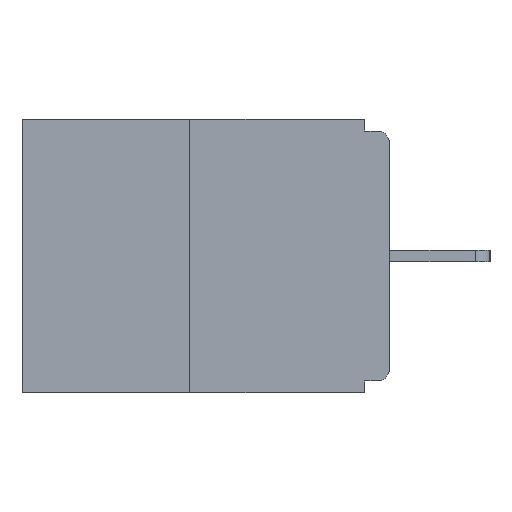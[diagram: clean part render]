
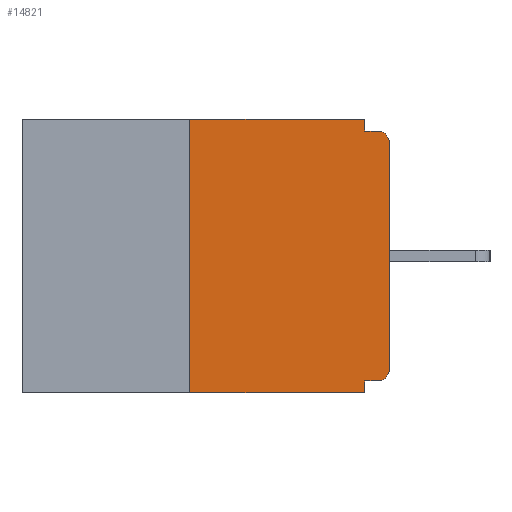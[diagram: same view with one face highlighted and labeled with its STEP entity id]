
A CAD part, left-side view. The second image highlights one B-rep face of the part: STEP entity #14821.
In plain terms, the highlighted planar face has unit normal (-1, 0, 0).
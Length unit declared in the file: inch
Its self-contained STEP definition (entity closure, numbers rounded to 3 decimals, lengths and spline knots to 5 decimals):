
#307 = VECTOR ( 'NONE', #3130, 39.37008 ) ;
#328 = LINE ( 'NONE', #7674, #12942 ) ;
#550 = DIRECTION ( 'NONE',  ( 1., 0., 0. ) ) ;
#706 = CARTESIAN_POINT ( 'NONE',  ( 0., 0.015, -0.015 ) ) ;
#743 = CIRCLE ( 'NONE', #5859, 0.015 ) ;
#1013 = VECTOR ( 'NONE', #22532, 39.37008 ) ;
#1101 = CARTESIAN_POINT ( 'NONE',  ( 0., 0., -0.03 ) ) ;
#1114 = DIRECTION ( 'NONE',  ( 0., 0., -1. ) ) ;
#1404 = CARTESIAN_POINT ( 'NONE',  ( 0., 0., -0.015 ) ) ;
#1560 = ORIENTED_EDGE ( 'NONE', *, *, #10027, .F. ) ;
#1850 = ORIENTED_EDGE ( 'NONE', *, *, #3985, .T. ) ;
#1979 = CARTESIAN_POINT ( 'NONE',  ( 0., 0.031, 0. ) ) ;
#2282 = CARTESIAN_POINT ( 'NONE',  ( 0., 0.46, 0. ) ) ;
#3026 = DIRECTION ( 'NONE',  ( 0., 0., -1. ) ) ;
#3130 = DIRECTION ( 'NONE',  ( 0., -1., 0. ) ) ;
#3823 = CIRCLE ( 'NONE', #12956, 0.015 ) ;
#3985 = EDGE_CURVE ( 'NONE', #8892, #7891, #743, .T. ) ;
#4742 = LINE ( 'NONE', #1404, #307 ) ;
#5058 = DIRECTION ( 'NONE',  ( 0., 0., 1. ) ) ;
#5859 = AXIS2_PLACEMENT_3D ( 'NONE', #19344, #10305, #22446 ) ;
#6465 = DIRECTION ( 'NONE',  ( 0., 0., -1. ) ) ;
#6553 = ORIENTED_EDGE ( 'NONE', *, *, #10595, .F. ) ;
#6658 = VERTEX_POINT ( 'NONE', #10700 ) ;
#7321 = EDGE_CURVE ( 'NONE', #12602, #14722, #8592, .T. ) ;
#7337 = CARTESIAN_POINT ( 'NONE',  ( 0., 0.031, 0. ) ) ;
#7428 = VECTOR ( 'NONE', #3026, 39.37008 ) ;
#7550 = ORIENTED_EDGE ( 'NONE', *, *, #7321, .T. ) ;
#7651 = EDGE_CURVE ( 'NONE', #12077, #7891, #4742, .T. ) ;
#7674 = CARTESIAN_POINT ( 'NONE',  ( 0., 0.46, 0. ) ) ;
#7891 = VERTEX_POINT ( 'NONE', #706 ) ;
#8220 = VERTEX_POINT ( 'NONE', #14110 ) ;
#8357 = CARTESIAN_POINT ( 'NONE',  ( 0., 0.46, -0.343 ) ) ;
#8382 = ORIENTED_EDGE ( 'NONE', *, *, #22657, .T. ) ;
#8491 = ORIENTED_EDGE ( 'NONE', *, *, #7651, .F. ) ;
#8592 = LINE ( 'NONE', #8357, #1013 ) ;
#8892 = VERTEX_POINT ( 'NONE', #1101 ) ;
#9675 = LINE ( 'NONE', #14958, #7428 ) ;
#9710 = DIRECTION ( 'NONE',  ( 0., 0., -1. ) ) ;
#9951 = LINE ( 'NONE', #17312, #18671 ) ;
#10015 = ORIENTED_EDGE ( 'NONE', *, *, #22618, .F. ) ;
#10027 = EDGE_CURVE ( 'NONE', #10649, #14722, #9675, .T. ) ;
#10154 = CARTESIAN_POINT ( 'NONE',  ( 0., 0.25, -0.343 ) ) ;
#10305 = DIRECTION ( 'NONE',  ( -1., 0., 0. ) ) ;
#10595 = EDGE_CURVE ( 'NONE', #6658, #10649, #20749, .T. ) ;
#10649 = VERTEX_POINT ( 'NONE', #17084 ) ;
#10700 = CARTESIAN_POINT ( 'NONE',  ( 0., 0.015, -0.328 ) ) ;
#10986 = FACE_OUTER_BOUND ( 'NONE', #12770, .T. ) ;
#11115 = DIRECTION ( 'NONE',  ( 0., -1., 0. ) ) ;
#11695 = DIRECTION ( 'NONE',  ( 0., 1., 0. ) ) ;
#12077 = VERTEX_POINT ( 'NONE', #16831 ) ;
#12139 = DIRECTION ( 'NONE',  ( 0., 0., 1. ) ) ;
#12190 = EDGE_CURVE ( 'NONE', #12602, #8220, #9951, .T. ) ;
#12298 = ORIENTED_EDGE ( 'NONE', *, *, #17455, .T. ) ;
#12602 = VERTEX_POINT ( 'NONE', #10154 ) ;
#12770 = EDGE_LOOP ( 'NONE', ( #10015, #16551, #7550, #1560, #6553, #8382, #12298, #1850, #8491, #15523 ) ) ;
#12928 = VECTOR ( 'NONE', #6465, 39.37008 ) ;
#12942 = VECTOR ( 'NONE', #11115, 39.37008 ) ;
#12956 = AXIS2_PLACEMENT_3D ( 'NONE', #14787, #18437, #9710 ) ;
#13066 = AXIS2_PLACEMENT_3D ( 'NONE', #2282, #550, #1114 ) ;
#13228 = VERTEX_POINT ( 'NONE', #19649 ) ;
#13278 = VECTOR ( 'NONE', #11695, 39.37008 ) ;
#14110 = CARTESIAN_POINT ( 'NONE',  ( 0., 0.25, 0. ) ) ;
#14722 = VERTEX_POINT ( 'NONE', #16494 ) ;
#14787 = CARTESIAN_POINT ( 'NONE',  ( 0., 0.015, -0.313 ) ) ;
#14821 = ADVANCED_FACE ( 'NONE', ( #10986 ), #17978, .F. ) ;
#14958 = CARTESIAN_POINT ( 'NONE',  ( 0., 0.031, -0.343 ) ) ;
#15523 = ORIENTED_EDGE ( 'NONE', *, *, #22097, .F. ) ;
#16033 = VERTEX_POINT ( 'NONE', #7337 ) ;
#16494 = CARTESIAN_POINT ( 'NONE',  ( 0., 0.031, -0.343 ) ) ;
#16551 = ORIENTED_EDGE ( 'NONE', *, *, #12190, .F. ) ;
#16831 = CARTESIAN_POINT ( 'NONE',  ( 0., 0.031, -0.015 ) ) ;
#17084 = CARTESIAN_POINT ( 'NONE',  ( 0., 0.031, -0.328 ) ) ;
#17312 = CARTESIAN_POINT ( 'NONE',  ( 0., 0.25, 0. ) ) ;
#17455 = EDGE_CURVE ( 'NONE', #13228, #8892, #18899, .T. ) ;
#17978 = PLANE ( 'NONE',  #13066 ) ;
#18437 = DIRECTION ( 'NONE',  ( -1., 0., 0. ) ) ;
#18671 = VECTOR ( 'NONE', #12139, 39.37008 ) ;
#18899 = LINE ( 'NONE', #19146, #19019 ) ;
#19019 = VECTOR ( 'NONE', #5058, 39.37008 ) ;
#19146 = CARTESIAN_POINT ( 'NONE',  ( 0., 0., 0. ) ) ;
#19344 = CARTESIAN_POINT ( 'NONE',  ( 0., 0.015, -0.03 ) ) ;
#19649 = CARTESIAN_POINT ( 'NONE',  ( 0., 0., -0.313 ) ) ;
#20749 = LINE ( 'NONE', #22565, #13278 ) ;
#22097 = EDGE_CURVE ( 'NONE', #16033, #12077, #22151, .T. ) ;
#22151 = LINE ( 'NONE', #1979, #12928 ) ;
#22446 = DIRECTION ( 'NONE',  ( 0., 0., -1. ) ) ;
#22532 = DIRECTION ( 'NONE',  ( 0., -1., 0. ) ) ;
#22565 = CARTESIAN_POINT ( 'NONE',  ( 0., 0., -0.328 ) ) ;
#22618 = EDGE_CURVE ( 'NONE', #8220, #16033, #328, .T. ) ;
#22657 = EDGE_CURVE ( 'NONE', #6658, #13228, #3823, .T. ) ;
